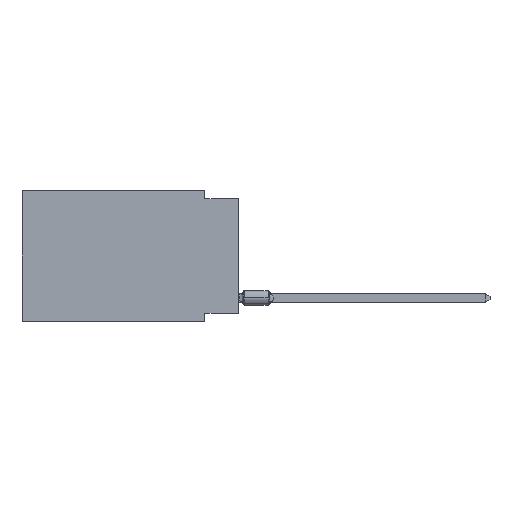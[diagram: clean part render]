
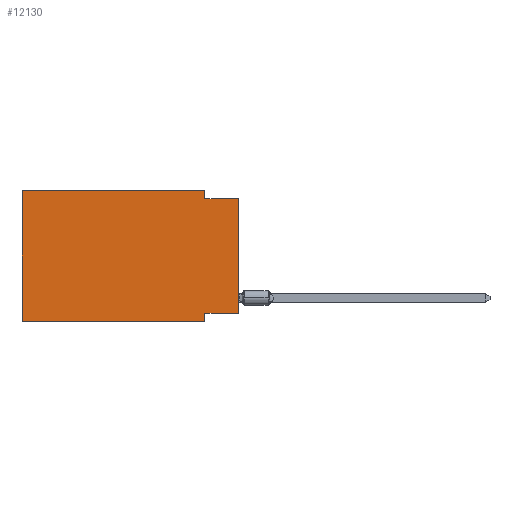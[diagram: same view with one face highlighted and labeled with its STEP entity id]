
A CAD part, left-side view. The second image highlights one B-rep face of the part: STEP entity #12130.
In plain terms, the highlighted planar face has unit normal (-1, 0, 0).
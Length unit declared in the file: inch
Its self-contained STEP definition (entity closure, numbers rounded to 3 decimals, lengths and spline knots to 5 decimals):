
#350 = ORIENTED_EDGE ( 'NONE', *, *, #4005, .F. ) ;
#750 = CARTESIAN_POINT ( 'NONE',  ( 0., 0.1, -0.025 ) ) ;
#1082 = PLANE ( 'NONE',  #4956 ) ;
#2072 = DIRECTION ( 'NONE',  ( 0., 0., -1. ) ) ;
#2102 = LINE ( 'NONE', #7878, #16582 ) ;
#2415 = LINE ( 'NONE', #8111, #14584 ) ;
#2436 = EDGE_CURVE ( 'NONE', #15764, #6252, #2415, .T. ) ;
#2638 = CARTESIAN_POINT ( 'NONE',  ( 0., 0.645, 0. ) ) ;
#2710 = LINE ( 'NONE', #4489, #7677 ) ;
#2979 = ORIENTED_EDGE ( 'NONE', *, *, #3069, .T. ) ;
#3061 = ORIENTED_EDGE ( 'NONE', *, *, #9589, .F. ) ;
#3069 = EDGE_CURVE ( 'NONE', #17997, #15865, #13115, .T. ) ;
#3625 = DIRECTION ( 'NONE',  ( 0., -1., 0. ) ) ;
#4005 = EDGE_CURVE ( 'NONE', #15213, #15865, #2710, .T. ) ;
#4115 = LINE ( 'NONE', #2638, #11810 ) ;
#4249 = VERTEX_POINT ( 'NONE', #8557 ) ;
#4489 = CARTESIAN_POINT ( 'NONE',  ( 0., 0., -0.025 ) ) ;
#4956 = AXIS2_PLACEMENT_3D ( 'NONE', #11623, #16294, #5758 ) ;
#5156 = EDGE_CURVE ( 'NONE', #15764, #4249, #4115, .T. ) ;
#5360 = EDGE_CURVE ( 'NONE', #6018, #15213, #2102, .T. ) ;
#5758 = DIRECTION ( 'NONE',  ( 0., 0., -1. ) ) ;
#6018 = VERTEX_POINT ( 'NONE', #9137 ) ;
#6247 = LINE ( 'NONE', #17074, #17906 ) ;
#6252 = VERTEX_POINT ( 'NONE', #9912 ) ;
#6300 = VECTOR ( 'NONE', #15214, 39.37008 ) ;
#6811 = DIRECTION ( 'NONE',  ( 0., -1., 0. ) ) ;
#7677 = VECTOR ( 'NONE', #14930, 39.37008 ) ;
#7878 = CARTESIAN_POINT ( 'NONE',  ( 0., 0.1, 0. ) ) ;
#7950 = ORIENTED_EDGE ( 'NONE', *, *, #18622, .F. ) ;
#8111 = CARTESIAN_POINT ( 'NONE',  ( 0., 0.645, -0.39 ) ) ;
#8339 = VECTOR ( 'NONE', #3625, 39.37008 ) ;
#8454 = DIRECTION ( 'NONE',  ( 0., 0., 1. ) ) ;
#8557 = CARTESIAN_POINT ( 'NONE',  ( 0., 0.645, 0. ) ) ;
#8712 = ORIENTED_EDGE ( 'NONE', *, *, #5360, .F. ) ;
#9137 = CARTESIAN_POINT ( 'NONE',  ( 0., 0.1, 0. ) ) ;
#9178 = LINE ( 'NONE', #16900, #6300 ) ;
#9589 = EDGE_CURVE ( 'NONE', #14576, #6252, #6247, .T. ) ;
#9912 = CARTESIAN_POINT ( 'NONE',  ( 0., 0.1, -0.39 ) ) ;
#10205 = CARTESIAN_POINT ( 'NONE',  ( 0., 0., -0.365 ) ) ;
#11623 = CARTESIAN_POINT ( 'NONE',  ( 0., 0.645, 0. ) ) ;
#11810 = VECTOR ( 'NONE', #19511, 39.37008 ) ;
#12130 = ADVANCED_FACE ( 'NONE', ( #17966 ), #1082, .F. ) ;
#12469 = LINE ( 'NONE', #18699, #8339 ) ;
#12624 = CARTESIAN_POINT ( 'NONE',  ( 0., 0.1, -0.365 ) ) ;
#13115 = LINE ( 'NONE', #17378, #19038 ) ;
#13859 = ORIENTED_EDGE ( 'NONE', *, *, #2436, .T. ) ;
#14488 = EDGE_CURVE ( 'NONE', #17997, #14576, #9178, .T. ) ;
#14576 = VERTEX_POINT ( 'NONE', #12624 ) ;
#14584 = VECTOR ( 'NONE', #6811, 39.37008 ) ;
#14921 = ORIENTED_EDGE ( 'NONE', *, *, #14488, .F. ) ;
#14930 = DIRECTION ( 'NONE',  ( 0., -1., 0. ) ) ;
#15072 = ORIENTED_EDGE ( 'NONE', *, *, #5156, .F. ) ;
#15213 = VERTEX_POINT ( 'NONE', #750 ) ;
#15214 = DIRECTION ( 'NONE',  ( 0., 1., 0. ) ) ;
#15716 = DIRECTION ( 'NONE',  ( 0., 0., -1. ) ) ;
#15764 = VERTEX_POINT ( 'NONE', #18603 ) ;
#15865 = VERTEX_POINT ( 'NONE', #18688 ) ;
#16294 = DIRECTION ( 'NONE',  ( 1., 0., 0. ) ) ;
#16546 = EDGE_LOOP ( 'NONE', ( #2979, #350, #8712, #7950, #15072, #13859, #3061, #14921 ) ) ;
#16582 = VECTOR ( 'NONE', #15716, 39.37008 ) ;
#16900 = CARTESIAN_POINT ( 'NONE',  ( 0., 0., -0.365 ) ) ;
#17074 = CARTESIAN_POINT ( 'NONE',  ( 0., 0.1, -0.39 ) ) ;
#17378 = CARTESIAN_POINT ( 'NONE',  ( 0., 0., 0. ) ) ;
#17906 = VECTOR ( 'NONE', #2072, 39.37008 ) ;
#17966 = FACE_OUTER_BOUND ( 'NONE', #16546, .T. ) ;
#17997 = VERTEX_POINT ( 'NONE', #10205 ) ;
#18603 = CARTESIAN_POINT ( 'NONE',  ( 0., 0.645, -0.39 ) ) ;
#18622 = EDGE_CURVE ( 'NONE', #4249, #6018, #12469, .T. ) ;
#18688 = CARTESIAN_POINT ( 'NONE',  ( 0., 0., -0.025 ) ) ;
#18699 = CARTESIAN_POINT ( 'NONE',  ( 0., 0.645, 0. ) ) ;
#19038 = VECTOR ( 'NONE', #8454, 39.37008 ) ;
#19511 = DIRECTION ( 'NONE',  ( 0., 0., 1. ) ) ;
